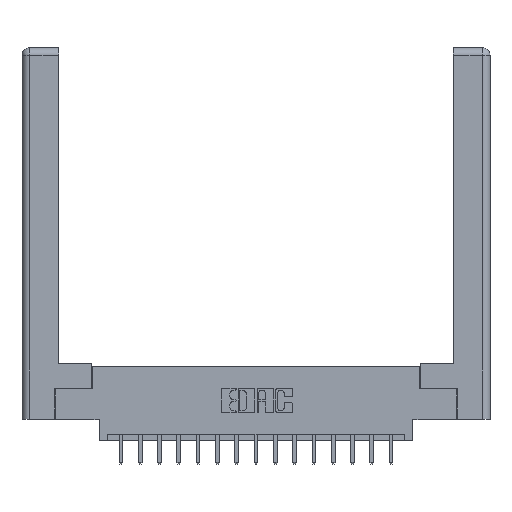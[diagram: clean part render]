
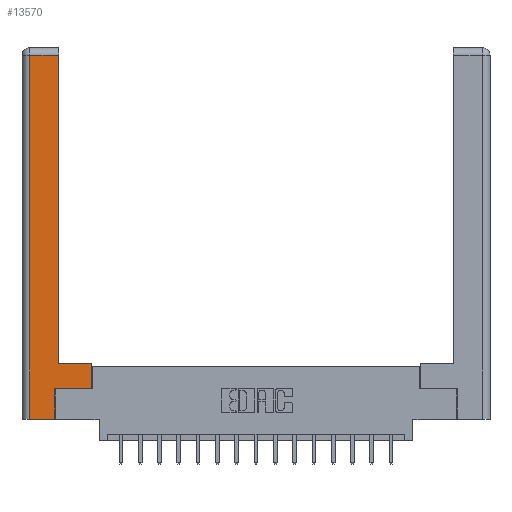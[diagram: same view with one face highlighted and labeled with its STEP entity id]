
A CAD part, top view. The second image highlights one B-rep face of the part: STEP entity #13570.
In plain terms, the highlighted planar face has unit normal (0, 0, 1).
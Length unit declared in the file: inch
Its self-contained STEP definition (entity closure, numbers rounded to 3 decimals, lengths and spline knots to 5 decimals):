
#59 = VERTEX_POINT ( 'NONE', #6025 ) ;
#958 = DIRECTION ( 'NONE',  ( -1., 0., 0. ) ) ;
#1264 = DIRECTION ( 'NONE',  ( 0., 1., 0. ) ) ;
#1532 = VERTEX_POINT ( 'NONE', #6119 ) ;
#1845 = DIRECTION ( 'NONE',  ( 1., 0., 0. ) ) ;
#2043 = VERTEX_POINT ( 'NONE', #2466 ) ;
#2118 = LINE ( 'NONE', #16373, #16502 ) ;
#2309 = VERTEX_POINT ( 'NONE', #4560 ) ;
#2387 = EDGE_CURVE ( 'NONE', #6154, #13143, #12761, .T. ) ;
#2466 = CARTESIAN_POINT ( 'NONE',  ( 0.0615, 2.94, 0. ) ) ;
#3157 = DIRECTION ( 'NONE',  ( 0., 1., 0. ) ) ;
#3648 = DIRECTION ( 'NONE',  ( 0., 0., -1. ) ) ;
#3961 = LINE ( 'NONE', #7049, #6185 ) ;
#4515 = CARTESIAN_POINT ( 'NONE',  ( 0.295, 3., 0. ) ) ;
#4521 = VECTOR ( 'NONE', #1845, 39.37008 ) ;
#4532 = EDGE_CURVE ( 'NONE', #1532, #2043, #15003, .T. ) ;
#4560 = CARTESIAN_POINT ( 'NONE',  ( 0.295, 0.45, 0. ) ) ;
#4620 = VECTOR ( 'NONE', #958, 39.37008 ) ;
#4804 = CARTESIAN_POINT ( 'NONE',  ( 0.265, 0., 0. ) ) ;
#4963 = EDGE_CURVE ( 'NONE', #2309, #1532, #5471, .T. ) ;
#5471 = LINE ( 'NONE', #4515, #6809 ) ;
#5515 = CARTESIAN_POINT ( 'NONE',  ( 0.565, 0.245, 0. ) ) ;
#5915 = CARTESIAN_POINT ( 'NONE',  ( 0.565, 0.245, 0. ) ) ;
#6025 = CARTESIAN_POINT ( 'NONE',  ( 0.265, 0.245, 0. ) ) ;
#6070 = CARTESIAN_POINT ( 'NONE',  ( 0.295, 0.45, 0. ) ) ;
#6119 = CARTESIAN_POINT ( 'NONE',  ( 0.295, 2.94, 0. ) ) ;
#6154 = VERTEX_POINT ( 'NONE', #11661 ) ;
#6163 = CARTESIAN_POINT ( 'NONE',  ( 0.265, 0., 0. ) ) ;
#6185 = VECTOR ( 'NONE', #1264, 39.37008 ) ;
#6809 = VECTOR ( 'NONE', #3157, 39.37008 ) ;
#7049 = CARTESIAN_POINT ( 'NONE',  ( 0.265, 0.245, 0. ) ) ;
#8106 = VECTOR ( 'NONE', #13780, 39.37008 ) ;
#8881 = EDGE_LOOP ( 'NONE', ( #11078, #15826, #14018, #9742, #13931, #16172, #9405, #14576 ) ) ;
#9202 = VECTOR ( 'NONE', #9732, 39.37008 ) ;
#9405 = ORIENTED_EDGE ( 'NONE', *, *, #17979, .T. ) ;
#9443 = DIRECTION ( 'NONE',  ( 0., 1., 0. ) ) ;
#9732 = DIRECTION ( 'NONE',  ( 1., 0., 0. ) ) ;
#9742 = ORIENTED_EDGE ( 'NONE', *, *, #2387, .T. ) ;
#9797 = EDGE_CURVE ( 'NONE', #13381, #2309, #17277, .T. ) ;
#9877 = VECTOR ( 'NONE', #15535, 39.37008 ) ;
#10504 = PLANE ( 'NONE',  #16727 ) ;
#10844 = FACE_OUTER_BOUND ( 'NONE', #8881, .T. ) ;
#10860 = EDGE_CURVE ( 'NONE', #59, #14383, #16579, .T. ) ;
#11078 = ORIENTED_EDGE ( 'NONE', *, *, #4963, .T. ) ;
#11617 = EDGE_CURVE ( 'NONE', #13143, #59, #3961, .T. ) ;
#11647 = EDGE_CURVE ( 'NONE', #2043, #6154, #13926, .T. ) ;
#11661 = CARTESIAN_POINT ( 'NONE',  ( 0.0615, 0., 0. ) ) ;
#12761 = LINE ( 'NONE', #4804, #4521 ) ;
#13143 = VERTEX_POINT ( 'NONE', #6163 ) ;
#13381 = VERTEX_POINT ( 'NONE', #16301 ) ;
#13570 = ADVANCED_FACE ( 'NONE', ( #10844 ), #10504, .F. ) ;
#13780 = DIRECTION ( 'NONE',  ( 0., -1., 0. ) ) ;
#13926 = LINE ( 'NONE', #15179, #8106 ) ;
#13931 = ORIENTED_EDGE ( 'NONE', *, *, #11617, .T. ) ;
#14018 = ORIENTED_EDGE ( 'NONE', *, *, #11647, .T. ) ;
#14383 = VERTEX_POINT ( 'NONE', #5915 ) ;
#14576 = ORIENTED_EDGE ( 'NONE', *, *, #9797, .T. ) ;
#15003 = LINE ( 'NONE', #17477, #4620 ) ;
#15179 = CARTESIAN_POINT ( 'NONE',  ( 0.0615, 0., 0. ) ) ;
#15535 = DIRECTION ( 'NONE',  ( -1., 0., 0. ) ) ;
#15826 = ORIENTED_EDGE ( 'NONE', *, *, #4532, .T. ) ;
#16088 = CARTESIAN_POINT ( 'NONE',  ( 0., 0., 0. ) ) ;
#16151 = DIRECTION ( 'NONE',  ( -1., 0., 0. ) ) ;
#16172 = ORIENTED_EDGE ( 'NONE', *, *, #10860, .T. ) ;
#16301 = CARTESIAN_POINT ( 'NONE',  ( 0.565, 0.45, 0. ) ) ;
#16373 = CARTESIAN_POINT ( 'NONE',  ( 0.565, 0.45, 0. ) ) ;
#16502 = VECTOR ( 'NONE', #9443, 39.37008 ) ;
#16579 = LINE ( 'NONE', #5515, #9202 ) ;
#16727 = AXIS2_PLACEMENT_3D ( 'NONE', #16088, #3648, #16151 ) ;
#17277 = LINE ( 'NONE', #6070, #9877 ) ;
#17477 = CARTESIAN_POINT ( 'NONE',  ( 0.0615, 2.94, 0. ) ) ;
#17979 = EDGE_CURVE ( 'NONE', #14383, #13381, #2118, .T. ) ;
